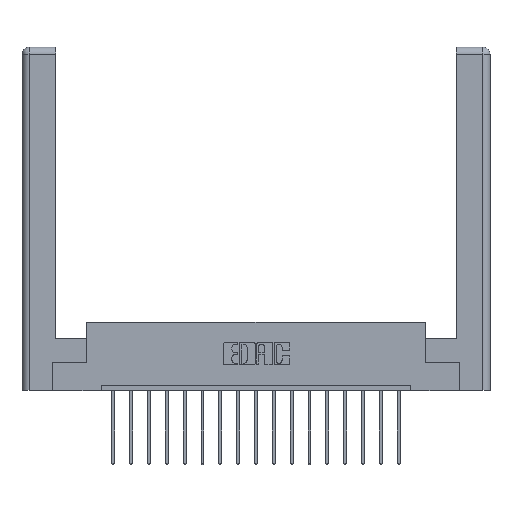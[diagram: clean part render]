
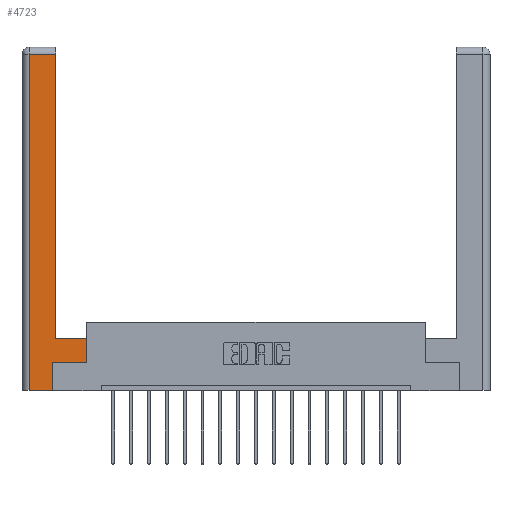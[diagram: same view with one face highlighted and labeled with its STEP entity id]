
A CAD part, top view. The second image highlights one B-rep face of the part: STEP entity #4723.
In plain terms, the highlighted planar face has unit normal (0, 0, 1).
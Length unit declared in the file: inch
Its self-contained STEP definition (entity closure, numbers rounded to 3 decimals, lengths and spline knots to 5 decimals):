
#111 = EDGE_LOOP ( 'NONE', ( #15329, #13726, #4676, #7172, #13152, #15440, #629, #13885 ) ) ;
#227 = CARTESIAN_POINT ( 'NONE',  ( 0.265, 0., 0. ) ) ;
#310 = VECTOR ( 'NONE', #17799, 39.37008 ) ;
#629 = ORIENTED_EDGE ( 'NONE', *, *, #13968, .T. ) ;
#993 = EDGE_CURVE ( 'NONE', #15215, #17100, #9500, .T. ) ;
#1899 = CARTESIAN_POINT ( 'NONE',  ( 0.565, 0.245, 0. ) ) ;
#2311 = CARTESIAN_POINT ( 'NONE',  ( 0.0615, 2.94, 0. ) ) ;
#2409 = CARTESIAN_POINT ( 'NONE',  ( 0., 0., 0. ) ) ;
#4380 = CARTESIAN_POINT ( 'NONE',  ( 0.565, 0.45, 0. ) ) ;
#4575 = DIRECTION ( 'NONE',  ( 0., 1., 0. ) ) ;
#4676 = ORIENTED_EDGE ( 'NONE', *, *, #16877, .T. ) ;
#4723 = ADVANCED_FACE ( 'NONE', ( #16048 ), #16738, .F. ) ;
#4964 = CARTESIAN_POINT ( 'NONE',  ( 0.265, 0.245, 0. ) ) ;
#5114 = DIRECTION ( 'NONE',  ( 0., 1., 0. ) ) ;
#5181 = EDGE_CURVE ( 'NONE', #10941, #14044, #6654, .T. ) ;
#5392 = VECTOR ( 'NONE', #7996, 39.37008 ) ;
#6633 = AXIS2_PLACEMENT_3D ( 'NONE', #2409, #13944, #13834 ) ;
#6654 = LINE ( 'NONE', #17793, #16937 ) ;
#6819 = VECTOR ( 'NONE', #14980, 39.37008 ) ;
#7172 = ORIENTED_EDGE ( 'NONE', *, *, #11790, .T. ) ;
#7252 = CARTESIAN_POINT ( 'NONE',  ( 0.0615, 0., 0. ) ) ;
#7324 = VECTOR ( 'NONE', #14866, 39.37008 ) ;
#7415 = EDGE_CURVE ( 'NONE', #17100, #12787, #15498, .T. ) ;
#7725 = VERTEX_POINT ( 'NONE', #11202 ) ;
#7996 = DIRECTION ( 'NONE',  ( -1., 0., 0. ) ) ;
#8072 = CARTESIAN_POINT ( 'NONE',  ( 0.295, 0.45, 0. ) ) ;
#8547 = CARTESIAN_POINT ( 'NONE',  ( 0.295, 0.45, 0. ) ) ;
#8781 = CARTESIAN_POINT ( 'NONE',  ( 0.265, 0.245, 0. ) ) ;
#9217 = CARTESIAN_POINT ( 'NONE',  ( 0.295, 3., 0. ) ) ;
#9258 = LINE ( 'NONE', #12083, #6819 ) ;
#9500 = LINE ( 'NONE', #9217, #11043 ) ;
#9555 = EDGE_CURVE ( 'NONE', #12167, #10941, #12006, .T. ) ;
#9630 = LINE ( 'NONE', #8072, #5392 ) ;
#9642 = LINE ( 'NONE', #4380, #16355 ) ;
#10941 = VERTEX_POINT ( 'NONE', #8781 ) ;
#11043 = VECTOR ( 'NONE', #5114, 39.37008 ) ;
#11202 = CARTESIAN_POINT ( 'NONE',  ( 0.565, 0.45, 0. ) ) ;
#11286 = CARTESIAN_POINT ( 'NONE',  ( 0.0615, 2.94, 0. ) ) ;
#11352 = DIRECTION ( 'NONE',  ( -1., 0., 0. ) ) ;
#11790 = EDGE_CURVE ( 'NONE', #18435, #12167, #9258, .T. ) ;
#12006 = LINE ( 'NONE', #4964, #7324 ) ;
#12022 = CARTESIAN_POINT ( 'NONE',  ( 0.0615, 0., 0. ) ) ;
#12083 = CARTESIAN_POINT ( 'NONE',  ( 0.265, 0., 0. ) ) ;
#12167 = VERTEX_POINT ( 'NONE', #227 ) ;
#12363 = LINE ( 'NONE', #12022, #310 ) ;
#12787 = VERTEX_POINT ( 'NONE', #2311 ) ;
#13152 = ORIENTED_EDGE ( 'NONE', *, *, #9555, .T. ) ;
#13726 = ORIENTED_EDGE ( 'NONE', *, *, #7415, .T. ) ;
#13834 = DIRECTION ( 'NONE',  ( -1., 0., 0. ) ) ;
#13885 = ORIENTED_EDGE ( 'NONE', *, *, #17910, .T. ) ;
#13944 = DIRECTION ( 'NONE',  ( 0., 0., -1. ) ) ;
#13968 = EDGE_CURVE ( 'NONE', #14044, #7725, #9642, .T. ) ;
#14044 = VERTEX_POINT ( 'NONE', #1899 ) ;
#14722 = DIRECTION ( 'NONE',  ( 1., 0., 0. ) ) ;
#14866 = DIRECTION ( 'NONE',  ( 0., 1., 0. ) ) ;
#14980 = DIRECTION ( 'NONE',  ( 1., 0., 0. ) ) ;
#15052 = VECTOR ( 'NONE', #11352, 39.37008 ) ;
#15215 = VERTEX_POINT ( 'NONE', #8547 ) ;
#15329 = ORIENTED_EDGE ( 'NONE', *, *, #993, .T. ) ;
#15440 = ORIENTED_EDGE ( 'NONE', *, *, #5181, .T. ) ;
#15498 = LINE ( 'NONE', #11286, #15052 ) ;
#16048 = FACE_OUTER_BOUND ( 'NONE', #111, .T. ) ;
#16355 = VECTOR ( 'NONE', #4575, 39.37008 ) ;
#16620 = CARTESIAN_POINT ( 'NONE',  ( 0.295, 2.94, 0. ) ) ;
#16738 = PLANE ( 'NONE',  #6633 ) ;
#16877 = EDGE_CURVE ( 'NONE', #12787, #18435, #12363, .T. ) ;
#16937 = VECTOR ( 'NONE', #14722, 39.37008 ) ;
#17100 = VERTEX_POINT ( 'NONE', #16620 ) ;
#17793 = CARTESIAN_POINT ( 'NONE',  ( 0.565, 0.245, 0. ) ) ;
#17799 = DIRECTION ( 'NONE',  ( 0., -1., 0. ) ) ;
#17910 = EDGE_CURVE ( 'NONE', #7725, #15215, #9630, .T. ) ;
#18435 = VERTEX_POINT ( 'NONE', #7252 ) ;
